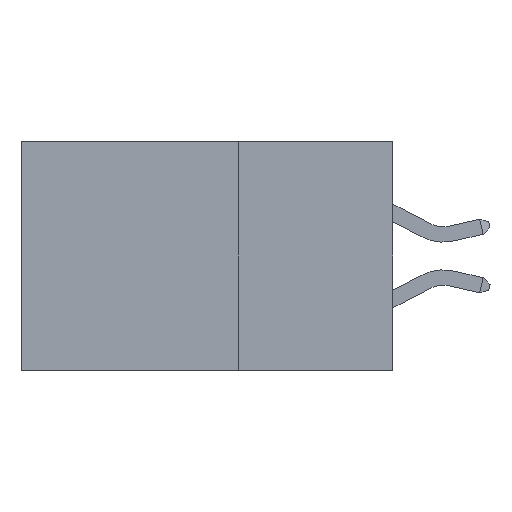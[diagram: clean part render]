
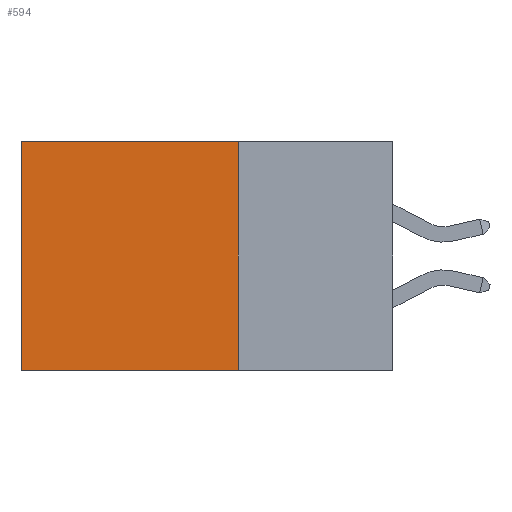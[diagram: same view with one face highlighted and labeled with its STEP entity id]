
A CAD part, left-side view. The second image highlights one B-rep face of the part: STEP entity #594.
In plain terms, the highlighted planar face has unit normal (-1, 0, 0).
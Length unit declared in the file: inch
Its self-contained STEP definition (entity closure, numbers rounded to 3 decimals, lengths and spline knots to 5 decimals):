
#594 = ADVANCED_FACE ( 'NONE', ( #15500 ), #15603, .F. ) ;
#924 = CARTESIAN_POINT ( 'NONE',  ( 0.2875, 0.6, 0. ) ) ;
#1426 = LINE ( 'NONE', #924, #6497 ) ;
#4654 = ORIENTED_EDGE ( 'NONE', *, *, #23431, .T. ) ;
#5475 = LINE ( 'NONE', #7061, #24375 ) ;
#5505 = CARTESIAN_POINT ( 'NONE',  ( 0.2875, 0.25, 0. ) ) ;
#5867 = ORIENTED_EDGE ( 'NONE', *, *, #15018, .T. ) ;
#6214 = VERTEX_POINT ( 'NONE', #25735 ) ;
#6497 = VECTOR ( 'NONE', #18278, 39.37008 ) ;
#6509 = CARTESIAN_POINT ( 'NONE',  ( 0.2875, 0.25, 0. ) ) ;
#6803 = DIRECTION ( 'NONE',  ( 0., 1., 0. ) ) ;
#7061 = CARTESIAN_POINT ( 'NONE',  ( 0.2875, 0.25, -0.37 ) ) ;
#7701 = ORIENTED_EDGE ( 'NONE', *, *, #31198, .F. ) ;
#9933 = CARTESIAN_POINT ( 'NONE',  ( 0.2875, 0.25, 0. ) ) ;
#10297 = AXIS2_PLACEMENT_3D ( 'NONE', #12881, #24869, #10413 ) ;
#10413 = DIRECTION ( 'NONE',  ( 0., 0., -1. ) ) ;
#10932 = ORIENTED_EDGE ( 'NONE', *, *, #16153, .F. ) ;
#12881 = CARTESIAN_POINT ( 'NONE',  ( 0.2875, 0.25, 0. ) ) ;
#14917 = VERTEX_POINT ( 'NONE', #21631 ) ;
#15018 = EDGE_CURVE ( 'NONE', #22016, #15860, #28513, .T. ) ;
#15500 = FACE_OUTER_BOUND ( 'NONE', #29015, .T. ) ;
#15603 = PLANE ( 'NONE',  #10297 ) ;
#15860 = VERTEX_POINT ( 'NONE', #17813 ) ;
#16153 = EDGE_CURVE ( 'NONE', #22016, #14917, #18094, .T. ) ;
#17747 = DIRECTION ( 'NONE',  ( 0., 1., 0. ) ) ;
#17813 = CARTESIAN_POINT ( 'NONE',  ( 0.2875, 0.6, 0. ) ) ;
#18094 = LINE ( 'NONE', #6509, #26138 ) ;
#18278 = DIRECTION ( 'NONE',  ( 0., 0., -1. ) ) ;
#20511 = VECTOR ( 'NONE', #17747, 39.37008 ) ;
#21631 = CARTESIAN_POINT ( 'NONE',  ( 0.2875, 0.25, -0.37 ) ) ;
#22016 = VERTEX_POINT ( 'NONE', #5505 ) ;
#23431 = EDGE_CURVE ( 'NONE', #15860, #6214, #1426, .T. ) ;
#24375 = VECTOR ( 'NONE', #6803, 39.37008 ) ;
#24869 = DIRECTION ( 'NONE',  ( 1., 0., 0. ) ) ;
#25735 = CARTESIAN_POINT ( 'NONE',  ( 0.2875, 0.6, -0.37 ) ) ;
#26138 = VECTOR ( 'NONE', #26928, 39.37008 ) ;
#26928 = DIRECTION ( 'NONE',  ( 0., 0., -1. ) ) ;
#28513 = LINE ( 'NONE', #9933, #20511 ) ;
#29015 = EDGE_LOOP ( 'NONE', ( #4654, #7701, #10932, #5867 ) ) ;
#31198 = EDGE_CURVE ( 'NONE', #14917, #6214, #5475, .T. ) ;
